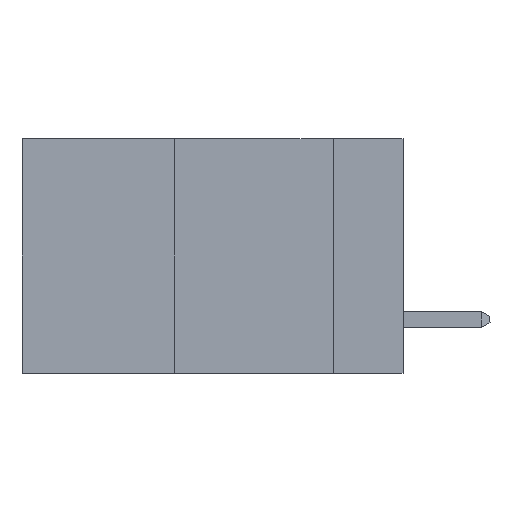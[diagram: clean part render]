
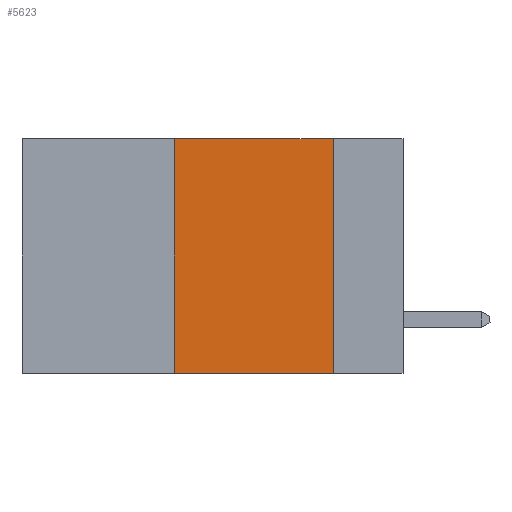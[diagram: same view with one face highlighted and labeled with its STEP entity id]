
A CAD part, left-side view. The second image highlights one B-rep face of the part: STEP entity #5623.
In plain terms, the highlighted planar face has unit normal (-1, 0, 0).
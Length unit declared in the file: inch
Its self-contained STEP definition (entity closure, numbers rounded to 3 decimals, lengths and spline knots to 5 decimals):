
#368 = EDGE_CURVE ( 'NONE', #6545, #1497, #9530, .T. ) ;
#758 = AXIS2_PLACEMENT_3D ( 'NONE', #9565, #4406, #11495 ) ;
#1497 = VERTEX_POINT ( 'NONE', #13108 ) ;
#1827 = DIRECTION ( 'NONE',  ( 0., -1., 0. ) ) ;
#2314 = CARTESIAN_POINT ( 'NONE',  ( 0., 0.11, 0. ) ) ;
#2371 = CARTESIAN_POINT ( 'NONE',  ( 0., 0.36, 0. ) ) ;
#3015 = LINE ( 'NONE', #6513, #5327 ) ;
#3156 = CARTESIAN_POINT ( 'NONE',  ( 0., 0.6, -0.37 ) ) ;
#3642 = FACE_OUTER_BOUND ( 'NONE', #5228, .T. ) ;
#4347 = DIRECTION ( 'NONE',  ( 0., -1., 0. ) ) ;
#4406 = DIRECTION ( 'NONE',  ( 1., 0., 0. ) ) ;
#4904 = VERTEX_POINT ( 'NONE', #7786 ) ;
#5137 = VECTOR ( 'NONE', #1827, 39.37008 ) ;
#5228 = EDGE_LOOP ( 'NONE', ( #10493, #8150, #10801, #13333 ) ) ;
#5327 = VECTOR ( 'NONE', #7513, 39.37008 ) ;
#5455 = PLANE ( 'NONE',  #758 ) ;
#5623 = ADVANCED_FACE ( 'NONE', ( #3642 ), #5455, .F. ) ;
#6500 = EDGE_CURVE ( 'NONE', #1497, #4904, #10290, .T. ) ;
#6513 = CARTESIAN_POINT ( 'NONE',  ( 0., 0.36, 0. ) ) ;
#6545 = VERTEX_POINT ( 'NONE', #2371 ) ;
#7513 = DIRECTION ( 'NONE',  ( 0., 0., 1. ) ) ;
#7601 = VECTOR ( 'NONE', #7798, 39.37008 ) ;
#7786 = CARTESIAN_POINT ( 'NONE',  ( 0., 0.11, -0.37 ) ) ;
#7798 = DIRECTION ( 'NONE',  ( 0., 0., -1. ) ) ;
#8150 = ORIENTED_EDGE ( 'NONE', *, *, #368, .F. ) ;
#9011 = EDGE_CURVE ( 'NONE', #11365, #6545, #3015, .T. ) ;
#9530 = LINE ( 'NONE', #13509, #11777 ) ;
#9565 = CARTESIAN_POINT ( 'NONE',  ( 0., 0.6, 0. ) ) ;
#10290 = LINE ( 'NONE', #2314, #7601 ) ;
#10493 = ORIENTED_EDGE ( 'NONE', *, *, #6500, .F. ) ;
#10521 = LINE ( 'NONE', #3156, #5137 ) ;
#10553 = EDGE_CURVE ( 'NONE', #11365, #4904, #10521, .T. ) ;
#10801 = ORIENTED_EDGE ( 'NONE', *, *, #9011, .F. ) ;
#11365 = VERTEX_POINT ( 'NONE', #13507 ) ;
#11495 = DIRECTION ( 'NONE',  ( 0., 0., -1. ) ) ;
#11777 = VECTOR ( 'NONE', #4347, 39.37008 ) ;
#13108 = CARTESIAN_POINT ( 'NONE',  ( 0., 0.11, 0. ) ) ;
#13333 = ORIENTED_EDGE ( 'NONE', *, *, #10553, .T. ) ;
#13507 = CARTESIAN_POINT ( 'NONE',  ( 0., 0.36, -0.37 ) ) ;
#13509 = CARTESIAN_POINT ( 'NONE',  ( 0., 0.6, 0. ) ) ;
